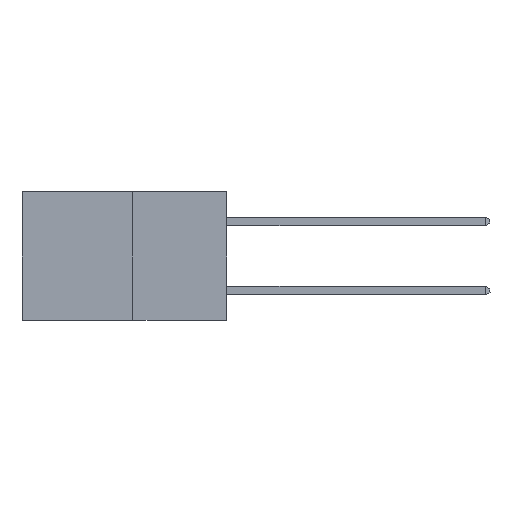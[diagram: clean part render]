
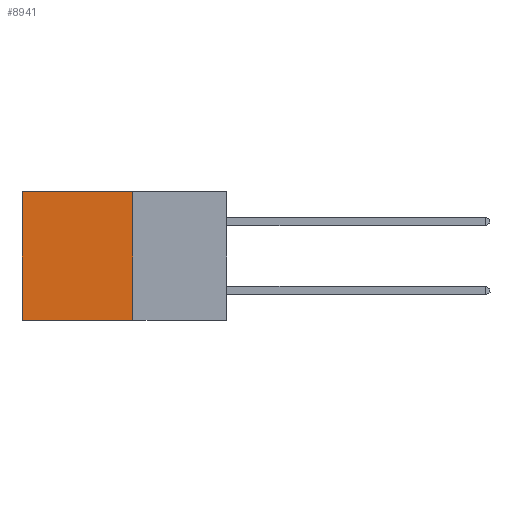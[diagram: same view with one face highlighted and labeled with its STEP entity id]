
A CAD part, left-side view. The second image highlights one B-rep face of the part: STEP entity #8941.
In plain terms, the highlighted planar face has unit normal (-1, 0, 0).
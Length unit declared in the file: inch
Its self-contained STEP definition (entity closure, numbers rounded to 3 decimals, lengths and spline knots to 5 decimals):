
#1062 = EDGE_LOOP ( 'NONE', ( #19425, #5618, #10168, #14026 ) ) ;
#2932 = CARTESIAN_POINT ( 'NONE',  ( 0.277, 0.59, -0.37 ) ) ;
#3757 = EDGE_CURVE ( 'NONE', #8165, #21286, #14871, .T. ) ;
#3799 = LINE ( 'NONE', #23186, #25533 ) ;
#4282 = LINE ( 'NONE', #6063, #20525 ) ;
#4637 = EDGE_CURVE ( 'NONE', #21286, #21334, #14818, .T. ) ;
#5362 = DIRECTION ( 'NONE',  ( 0., 1., 0. ) ) ;
#5618 = ORIENTED_EDGE ( 'NONE', *, *, #20530, .F. ) ;
#6063 = CARTESIAN_POINT ( 'NONE',  ( 0.277, 0.27, -0.37 ) ) ;
#6278 = CARTESIAN_POINT ( 'NONE',  ( 0.277, 0.27, 0. ) ) ;
#7290 = DIRECTION ( 'NONE',  ( 0., 0., -1. ) ) ;
#7317 = DIRECTION ( 'NONE',  ( 1., 0., 0. ) ) ;
#7356 = CARTESIAN_POINT ( 'NONE',  ( 0.277, 0.27, -0.37 ) ) ;
#7383 = CARTESIAN_POINT ( 'NONE',  ( 0.277, 0.27, -0.37 ) ) ;
#7728 = PLANE ( 'NONE',  #9219 ) ;
#8165 = VERTEX_POINT ( 'NONE', #25925 ) ;
#8941 = ADVANCED_FACE ( 'NONE', ( #17290 ), #7728, .F. ) ;
#9219 = AXIS2_PLACEMENT_3D ( 'NONE', #7356, #7317, #7290 ) ;
#10168 = ORIENTED_EDGE ( 'NONE', *, *, #27046, .F. ) ;
#14026 = ORIENTED_EDGE ( 'NONE', *, *, #3757, .T. ) ;
#14818 = LINE ( 'NONE', #15578, #25216 ) ;
#14871 = LINE ( 'NONE', #6278, #19105 ) ;
#15578 = CARTESIAN_POINT ( 'NONE',  ( 0.277, 0.59, -0.37 ) ) ;
#15666 = DIRECTION ( 'NONE',  ( 0., 0., -1. ) ) ;
#16999 = DIRECTION ( 'NONE',  ( 0., 1., 0. ) ) ;
#17290 = FACE_OUTER_BOUND ( 'NONE', #1062, .T. ) ;
#19105 = VECTOR ( 'NONE', #5362, 39.37008 ) ;
#19425 = ORIENTED_EDGE ( 'NONE', *, *, #4637, .T. ) ;
#19712 = CARTESIAN_POINT ( 'NONE',  ( 0.277, 0.59, 0. ) ) ;
#20525 = VECTOR ( 'NONE', #22909, 39.37008 ) ;
#20530 = EDGE_CURVE ( 'NONE', #20731, #21334, #3799, .T. ) ;
#20731 = VERTEX_POINT ( 'NONE', #7383 ) ;
#21286 = VERTEX_POINT ( 'NONE', #19712 ) ;
#21334 = VERTEX_POINT ( 'NONE', #2932 ) ;
#22909 = DIRECTION ( 'NONE',  ( 0., 0., -1. ) ) ;
#23186 = CARTESIAN_POINT ( 'NONE',  ( 0.277, 0.27, -0.37 ) ) ;
#25216 = VECTOR ( 'NONE', #15666, 39.37008 ) ;
#25533 = VECTOR ( 'NONE', #16999, 39.37008 ) ;
#25925 = CARTESIAN_POINT ( 'NONE',  ( 0.277, 0.27, 0. ) ) ;
#27046 = EDGE_CURVE ( 'NONE', #8165, #20731, #4282, .T. ) ;
